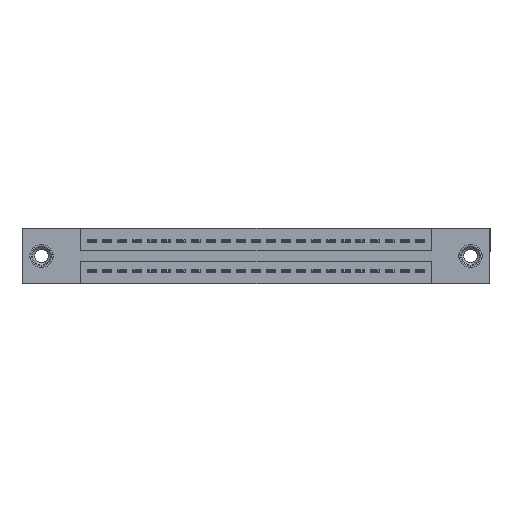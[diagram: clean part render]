
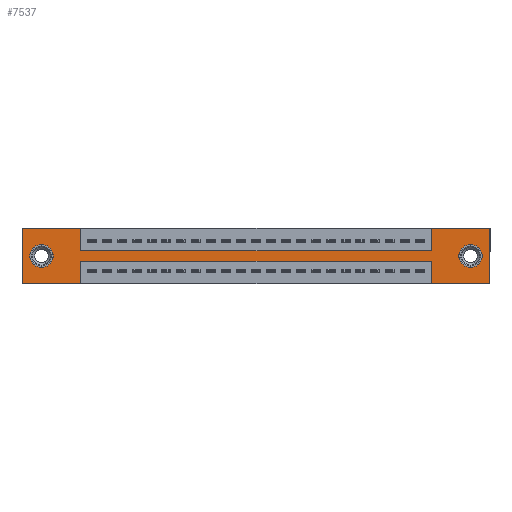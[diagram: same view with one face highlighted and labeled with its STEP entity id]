
A CAD part, front view. The second image highlights one B-rep face of the part: STEP entity #7537.
In plain terms, the highlighted planar face has unit normal (0, -1, 0).
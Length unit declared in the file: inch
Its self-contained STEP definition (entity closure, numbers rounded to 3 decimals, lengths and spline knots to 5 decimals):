
#19 = ORIENTED_EDGE ( 'NONE', *, *, #20943, .F. ) ;
#350 = DIRECTION ( 'NONE',  ( 1., 0., 0. ) ) ;
#777 = CARTESIAN_POINT ( 'NONE',  ( 0.13, 0., -0.107 ) ) ;
#1031 = CARTESIAN_POINT ( 'NONE',  ( 3.135, 0., 0. ) ) ;
#1143 = DIRECTION ( 'NONE',  ( 0., 1., 0. ) ) ;
#1228 = EDGE_LOOP ( 'NONE', ( #7985, #13573, #19, #8691, #4887, #22373, #17919, #18865, #4886, #14003, #6749, #12165 ) ) ;
#1275 = CIRCLE ( 'NONE', #13223, 0.078 ) ;
#1437 = DIRECTION ( 'NONE',  ( 0., 0., -1. ) ) ;
#1439 = CARTESIAN_POINT ( 'NONE',  ( 3.135, 0., 0. ) ) ;
#1455 = CIRCLE ( 'NONE', #12865, 0.078 ) ;
#1556 = DIRECTION ( 'NONE',  ( 0., 1., 0. ) ) ;
#1988 = CARTESIAN_POINT ( 'NONE',  ( 0., 0., 0. ) ) ;
#2754 = EDGE_CURVE ( 'NONE', #18679, #14086, #21098, .T. ) ;
#2807 = DIRECTION ( 'NONE',  ( 0., 1., 0. ) ) ;
#2850 = CARTESIAN_POINT ( 'NONE',  ( 0.3925, 0., -0.22 ) ) ;
#2930 = CARTESIAN_POINT ( 'NONE',  ( 3.005, 0., -0.107 ) ) ;
#3393 = VECTOR ( 'NONE', #350, 39.37008 ) ;
#3603 = EDGE_CURVE ( 'NONE', #11033, #6818, #1455, .T. ) ;
#3654 = LINE ( 'NONE', #6493, #20988 ) ;
#3864 = DIRECTION ( 'NONE',  ( 0., 0., 1. ) ) ;
#3937 = VERTEX_POINT ( 'NONE', #12700 ) ;
#4473 = VERTEX_POINT ( 'NONE', #10660 ) ;
#4886 = ORIENTED_EDGE ( 'NONE', *, *, #7916, .F. ) ;
#4887 = ORIENTED_EDGE ( 'NONE', *, *, #17852, .F. ) ;
#5231 = LINE ( 'NONE', #14535, #9431 ) ;
#5562 = CARTESIAN_POINT ( 'NONE',  ( 3.135, 0., -0.37 ) ) ;
#5848 = DIRECTION ( 'NONE',  ( 0., 0., 1. ) ) ;
#6245 = EDGE_LOOP ( 'NONE', ( #8026, #9424 ) ) ;
#6272 = VERTEX_POINT ( 'NONE', #1031 ) ;
#6493 = CARTESIAN_POINT ( 'NONE',  ( 0.3925, 0., -0.15 ) ) ;
#6606 = VERTEX_POINT ( 'NONE', #19535 ) ;
#6728 = EDGE_CURVE ( 'NONE', #13477, #9325, #7481, .T. ) ;
#6749 = ORIENTED_EDGE ( 'NONE', *, *, #20260, .F. ) ;
#6818 = VERTEX_POINT ( 'NONE', #21767 ) ;
#6961 = CARTESIAN_POINT ( 'NONE',  ( 0.13, 0., -0.263 ) ) ;
#7252 = CARTESIAN_POINT ( 'NONE',  ( 3.005, 0., -0.185 ) ) ;
#7357 = VECTOR ( 'NONE', #1437, 39.37008 ) ;
#7481 = LINE ( 'NONE', #21528, #11647 ) ;
#7537 = ADVANCED_FACE ( 'NONE', ( #21709, #8574, #14266 ), #18478, .T. ) ;
#7591 = DIRECTION ( 'NONE',  ( -1., 0., 0. ) ) ;
#7660 = EDGE_CURVE ( 'NONE', #14979, #18679, #19564, .T. ) ;
#7916 = EDGE_CURVE ( 'NONE', #9325, #6606, #10791, .T. ) ;
#7985 = ORIENTED_EDGE ( 'NONE', *, *, #2754, .F. ) ;
#8026 = ORIENTED_EDGE ( 'NONE', *, *, #3603, .T. ) ;
#8028 = LINE ( 'NONE', #12691, #16675 ) ;
#8221 = CARTESIAN_POINT ( 'NONE',  ( 0.3925, 0., -0.37 ) ) ;
#8388 = CARTESIAN_POINT ( 'NONE',  ( 0.3925, 0., -0.22 ) ) ;
#8428 = CARTESIAN_POINT ( 'NONE',  ( 0., 0., -0.37 ) ) ;
#8574 = FACE_BOUND ( 'NONE', #22431, .T. ) ;
#8691 = ORIENTED_EDGE ( 'NONE', *, *, #20612, .F. ) ;
#8696 = CARTESIAN_POINT ( 'NONE',  ( 2.7425, 0., -0.22 ) ) ;
#9010 = EDGE_CURVE ( 'NONE', #16750, #12088, #10521, .T. ) ;
#9077 = DIRECTION ( 'NONE',  ( 0., 0., -1. ) ) ;
#9158 = CARTESIAN_POINT ( 'NONE',  ( 0., 0., -0.37 ) ) ;
#9323 = CARTESIAN_POINT ( 'NONE',  ( 0., 0., 0. ) ) ;
#9325 = VERTEX_POINT ( 'NONE', #21358 ) ;
#9424 = ORIENTED_EDGE ( 'NONE', *, *, #20201, .T. ) ;
#9431 = VECTOR ( 'NONE', #5848, 39.37008 ) ;
#9624 = VERTEX_POINT ( 'NONE', #19967 ) ;
#9713 = CARTESIAN_POINT ( 'NONE',  ( 0., 0., 0. ) ) ;
#9733 = VECTOR ( 'NONE', #18724, 39.37008 ) ;
#9969 = CARTESIAN_POINT ( 'NONE',  ( 0., 0., -0.37 ) ) ;
#9989 = CARTESIAN_POINT ( 'NONE',  ( 0.3925, 0., -0.37 ) ) ;
#10126 = EDGE_CURVE ( 'NONE', #14086, #18349, #16340, .T. ) ;
#10366 = ORIENTED_EDGE ( 'NONE', *, *, #9010, .T. ) ;
#10518 = VECTOR ( 'NONE', #11918, 39.37008 ) ;
#10521 = CIRCLE ( 'NONE', #17419, 0.078 ) ;
#10660 = CARTESIAN_POINT ( 'NONE',  ( 2.7425, 0., 0. ) ) ;
#10684 = VERTEX_POINT ( 'NONE', #5562 ) ;
#10791 = LINE ( 'NONE', #17643, #14248 ) ;
#11033 = VERTEX_POINT ( 'NONE', #2930 ) ;
#11596 = AXIS2_PLACEMENT_3D ( 'NONE', #7252, #19331, #9077 ) ;
#11647 = VECTOR ( 'NONE', #13078, 39.37008 ) ;
#11707 = DIRECTION ( 'NONE',  ( 0., 0., -1. ) ) ;
#11819 = CARTESIAN_POINT ( 'NONE',  ( 3.005, 0., -0.185 ) ) ;
#11918 = DIRECTION ( 'NONE',  ( -1., 0., 0. ) ) ;
#12075 = DIRECTION ( 'NONE',  ( 0., 0., -1. ) ) ;
#12088 = VERTEX_POINT ( 'NONE', #777 ) ;
#12165 = ORIENTED_EDGE ( 'NONE', *, *, #10126, .F. ) ;
#12169 = CARTESIAN_POINT ( 'NONE',  ( 0.13, 0., -0.185 ) ) ;
#12691 = CARTESIAN_POINT ( 'NONE',  ( 2.7425, 0., -0.37 ) ) ;
#12700 = CARTESIAN_POINT ( 'NONE',  ( 2.7425, 0., -0.15 ) ) ;
#12865 = AXIS2_PLACEMENT_3D ( 'NONE', #11819, #1143, #13535 ) ;
#13078 = DIRECTION ( 'NONE',  ( 1., 0., 0. ) ) ;
#13223 = AXIS2_PLACEMENT_3D ( 'NONE', #13338, #2807, #15062 ) ;
#13332 = EDGE_CURVE ( 'NONE', #4473, #6272, #17272, .T. ) ;
#13338 = CARTESIAN_POINT ( 'NONE',  ( 0.13, 0., -0.185 ) ) ;
#13477 = VERTEX_POINT ( 'NONE', #9713 ) ;
#13535 = DIRECTION ( 'NONE',  ( 0., 0., -1. ) ) ;
#13573 = ORIENTED_EDGE ( 'NONE', *, *, #7660, .F. ) ;
#13599 = EDGE_CURVE ( 'NONE', #6606, #3937, #3654, .T. ) ;
#13889 = DIRECTION ( 'NONE',  ( 0., 0., 1. ) ) ;
#14003 = ORIENTED_EDGE ( 'NONE', *, *, #6728, .F. ) ;
#14086 = VERTEX_POINT ( 'NONE', #9989 ) ;
#14248 = VECTOR ( 'NONE', #19341, 39.37008 ) ;
#14266 = FACE_OUTER_BOUND ( 'NONE', #1228, .T. ) ;
#14298 = CIRCLE ( 'NONE', #11596, 0.078 ) ;
#14535 = CARTESIAN_POINT ( 'NONE',  ( 2.7425, 0., 0. ) ) ;
#14566 = EDGE_CURVE ( 'NONE', #3937, #4473, #5231, .T. ) ;
#14769 = EDGE_CURVE ( 'NONE', #12088, #16750, #1275, .T. ) ;
#14979 = VERTEX_POINT ( 'NONE', #8696 ) ;
#15062 = DIRECTION ( 'NONE',  ( 0., 0., 1. ) ) ;
#16186 = DIRECTION ( 'NONE',  ( 0., 0., 1. ) ) ;
#16340 = LINE ( 'NONE', #17952, #20331 ) ;
#16675 = VECTOR ( 'NONE', #16186, 39.37008 ) ;
#16750 = VERTEX_POINT ( 'NONE', #6961 ) ;
#16877 = DIRECTION ( 'NONE',  ( 1., 0., 0. ) ) ;
#17064 = LINE ( 'NONE', #1439, #22118 ) ;
#17272 = LINE ( 'NONE', #9323, #3393 ) ;
#17419 = AXIS2_PLACEMENT_3D ( 'NONE', #12169, #1556, #13889 ) ;
#17643 = CARTESIAN_POINT ( 'NONE',  ( 0.3925, 0., 0. ) ) ;
#17767 = LINE ( 'NONE', #1988, #22272 ) ;
#17852 = EDGE_CURVE ( 'NONE', #6272, #10684, #17064, .T. ) ;
#17919 = ORIENTED_EDGE ( 'NONE', *, *, #14566, .F. ) ;
#17952 = CARTESIAN_POINT ( 'NONE',  ( 0., 0., -0.37 ) ) ;
#18274 = LINE ( 'NONE', #8428, #9733 ) ;
#18349 = VERTEX_POINT ( 'NONE', #9158 ) ;
#18478 = PLANE ( 'NONE',  #20251 ) ;
#18679 = VERTEX_POINT ( 'NONE', #2850 ) ;
#18724 = DIRECTION ( 'NONE',  ( -1., 0., 0. ) ) ;
#18865 = ORIENTED_EDGE ( 'NONE', *, *, #13599, .F. ) ;
#19331 = DIRECTION ( 'NONE',  ( 0., 1., 0. ) ) ;
#19341 = DIRECTION ( 'NONE',  ( 0., 0., -1. ) ) ;
#19535 = CARTESIAN_POINT ( 'NONE',  ( 0.3925, 0., -0.15 ) ) ;
#19564 = LINE ( 'NONE', #8388, #10518 ) ;
#19885 = ORIENTED_EDGE ( 'NONE', *, *, #14769, .T. ) ;
#19967 = CARTESIAN_POINT ( 'NONE',  ( 2.7425, 0., -0.37 ) ) ;
#20201 = EDGE_CURVE ( 'NONE', #6818, #11033, #14298, .T. ) ;
#20251 = AXIS2_PLACEMENT_3D ( 'NONE', #9969, #21884, #11707 ) ;
#20260 = EDGE_CURVE ( 'NONE', #18349, #13477, #17767, .T. ) ;
#20331 = VECTOR ( 'NONE', #7591, 39.37008 ) ;
#20612 = EDGE_CURVE ( 'NONE', #10684, #9624, #18274, .T. ) ;
#20943 = EDGE_CURVE ( 'NONE', #9624, #14979, #8028, .T. ) ;
#20988 = VECTOR ( 'NONE', #16877, 39.37008 ) ;
#21098 = LINE ( 'NONE', #8221, #7357 ) ;
#21358 = CARTESIAN_POINT ( 'NONE',  ( 0.3925, 0., 0. ) ) ;
#21528 = CARTESIAN_POINT ( 'NONE',  ( 0., 0., 0. ) ) ;
#21709 = FACE_BOUND ( 'NONE', #6245, .T. ) ;
#21767 = CARTESIAN_POINT ( 'NONE',  ( 3.005, 0., -0.263 ) ) ;
#21884 = DIRECTION ( 'NONE',  ( 0., -1., 0. ) ) ;
#22118 = VECTOR ( 'NONE', #12075, 39.37008 ) ;
#22272 = VECTOR ( 'NONE', #3864, 39.37008 ) ;
#22373 = ORIENTED_EDGE ( 'NONE', *, *, #13332, .F. ) ;
#22431 = EDGE_LOOP ( 'NONE', ( #19885, #10366 ) ) ;
